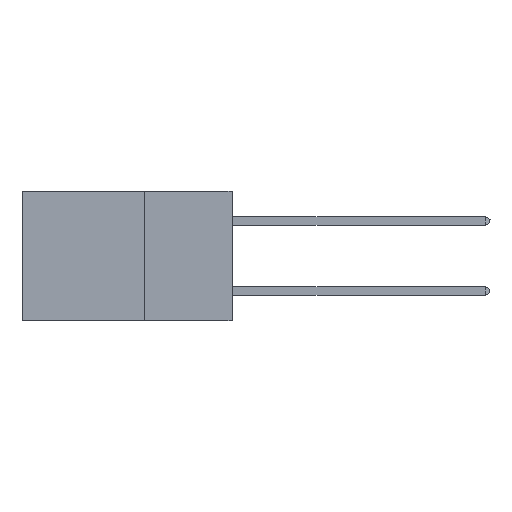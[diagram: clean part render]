
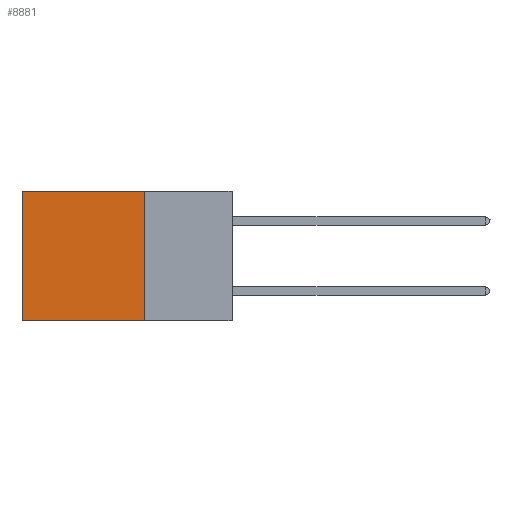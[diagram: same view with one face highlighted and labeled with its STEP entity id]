
A CAD part, left-side view. The second image highlights one B-rep face of the part: STEP entity #8881.
In plain terms, the highlighted planar face has unit normal (-1, 0, 0).
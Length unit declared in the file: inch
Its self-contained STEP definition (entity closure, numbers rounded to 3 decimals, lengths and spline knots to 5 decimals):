
#30 = ORIENTED_EDGE ( 'NONE', *, *, #24691, .T. ) ;
#276 = CARTESIAN_POINT ( 'NONE',  ( 0.2875, 0.25, -0.37 ) ) ;
#635 = EDGE_CURVE ( 'NONE', #9693, #12101, #14540, .T. ) ;
#930 = VECTOR ( 'NONE', #7720, 39.37008 ) ;
#2022 = AXIS2_PLACEMENT_3D ( 'NONE', #9631, #24208, #11769 ) ;
#2250 = DIRECTION ( 'NONE',  ( 0., 1., 0. ) ) ;
#2691 = DIRECTION ( 'NONE',  ( 0., 1., 0. ) ) ;
#2942 = ORIENTED_EDGE ( 'NONE', *, *, #19142, .F. ) ;
#4398 = CARTESIAN_POINT ( 'NONE',  ( 0.2875, 0.25, 0. ) ) ;
#5324 = PLANE ( 'NONE',  #2022 ) ;
#5375 = VERTEX_POINT ( 'NONE', #19692 ) ;
#6292 = DIRECTION ( 'NONE',  ( 0., 0., -1. ) ) ;
#6771 = CARTESIAN_POINT ( 'NONE',  ( 0.2875, 0.6, 0. ) ) ;
#7482 = EDGE_CURVE ( 'NONE', #14109, #12101, #13463, .T. ) ;
#7720 = DIRECTION ( 'NONE',  ( 0., 0., -1. ) ) ;
#8180 = CARTESIAN_POINT ( 'NONE',  ( 0.2875, 0.6, 0. ) ) ;
#8881 = ADVANCED_FACE ( 'NONE', ( #9921 ), #5324, .F. ) ;
#8919 = VECTOR ( 'NONE', #6292, 39.37008 ) ;
#9631 = CARTESIAN_POINT ( 'NONE',  ( 0.2875, 0.25, 0. ) ) ;
#9693 = VERTEX_POINT ( 'NONE', #8180 ) ;
#9758 = CARTESIAN_POINT ( 'NONE',  ( 0.2875, 0.6, -0.37 ) ) ;
#9921 = FACE_OUTER_BOUND ( 'NONE', #18463, .T. ) ;
#11769 = DIRECTION ( 'NONE',  ( 0., 0., -1. ) ) ;
#12101 = VERTEX_POINT ( 'NONE', #9758 ) ;
#12808 = VECTOR ( 'NONE', #2691, 39.37008 ) ;
#13463 = LINE ( 'NONE', #19612, #12808 ) ;
#14109 = VERTEX_POINT ( 'NONE', #276 ) ;
#14302 = VECTOR ( 'NONE', #2250, 39.37008 ) ;
#14540 = LINE ( 'NONE', #6771, #8919 ) ;
#17150 = LINE ( 'NONE', #20331, #930 ) ;
#18463 = EDGE_LOOP ( 'NONE', ( #23656, #24439, #2942, #30 ) ) ;
#19142 = EDGE_CURVE ( 'NONE', #5375, #14109, #17150, .T. ) ;
#19612 = CARTESIAN_POINT ( 'NONE',  ( 0.2875, 0.25, -0.37 ) ) ;
#19692 = CARTESIAN_POINT ( 'NONE',  ( 0.2875, 0.25, 0. ) ) ;
#20331 = CARTESIAN_POINT ( 'NONE',  ( 0.2875, 0.25, 0. ) ) ;
#20496 = LINE ( 'NONE', #4398, #14302 ) ;
#23656 = ORIENTED_EDGE ( 'NONE', *, *, #635, .T. ) ;
#24208 = DIRECTION ( 'NONE',  ( 1., 0., 0. ) ) ;
#24439 = ORIENTED_EDGE ( 'NONE', *, *, #7482, .F. ) ;
#24691 = EDGE_CURVE ( 'NONE', #5375, #9693, #20496, .T. ) ;
